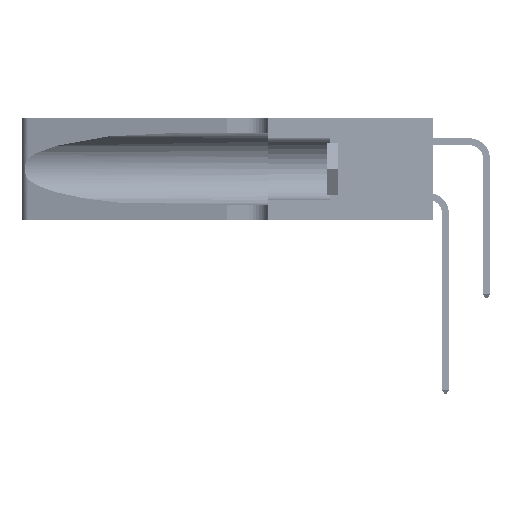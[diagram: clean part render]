
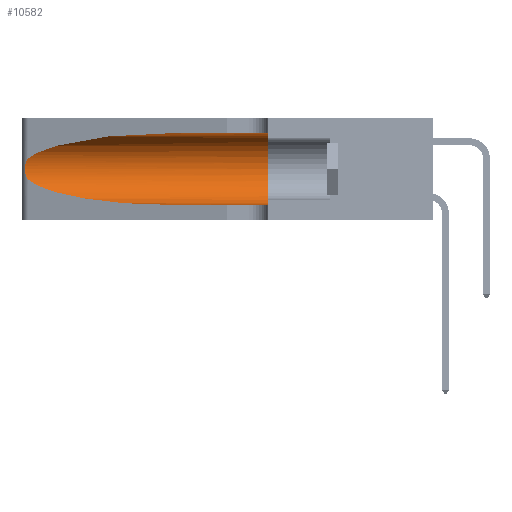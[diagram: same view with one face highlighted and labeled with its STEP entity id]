
A CAD part, left-side view. The second image highlights one B-rep face of the part: STEP entity #10582.
In plain terms, the highlighted cylindrical face has radius 3.308 mm (diameter 6.617 mm), a partial arc.
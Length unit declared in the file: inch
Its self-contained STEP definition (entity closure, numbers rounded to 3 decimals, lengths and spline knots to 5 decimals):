
#1970 = CARTESIAN_POINT ( 'NONE',  ( 0.1305, 1.61858, 0.05475 ) ) ;
#4043 = CARTESIAN_POINT ( 'NONE',  ( 0.25854, 1.2359, 0.20912 ) ) ;
#6457 = CARTESIAN_POINT ( 'NONE',  ( 0.1305, 0.72297, 0.31525 ) ) ;
#7393 = VECTOR ( 'NONE', #19006, 39.37008 ) ;
#8060 = FACE_OUTER_BOUND ( 'NONE', #13091, .T. ) ;
#8213 = CARTESIAN_POINT ( 'NONE',  ( 0.26075, 1.23896, 0.19203 ) ) ;
#8369 = ORIENTED_EDGE ( 'NONE', *, *, #14442, .T. ) ;
#10315 = CARTESIAN_POINT ( 'NONE',  ( 0.1305, 0.35, 0.185 ) ) ;
#10350 = DIRECTION ( 'NONE',  ( 0., -1., 0. ) ) ;
#10582 = ADVANCED_FACE ( 'NONE', ( #8060 ), #17905, .F. ) ;
#11391 = ORIENTED_EDGE ( 'NONE', *, *, #20961, .F. ) ;
#12233 = CARTESIAN_POINT ( 'NONE',  ( 0.25487, 1.22718, 0.22369 ) ) ;
#12414 = CARTESIAN_POINT ( 'NONE',  ( 0.26017, 1.23833, 0.17102 ) ) ;
#12595 = CARTESIAN_POINT ( 'NONE',  ( 0.1305, 0.72297, 0.31525 ) ) ;
#13091 = EDGE_LOOP ( 'NONE', ( #46398, #51525, #8369, #25007, #44437, #11391 ) ) ;
#14442 = EDGE_CURVE ( 'NONE', #21079, #15864, #38820, .T. ) ;
#14537 = DIRECTION ( 'NONE',  ( 0., 0., 1. ) ) ;
#15864 = VERTEX_POINT ( 'NONE', #43394 ) ;
#16449 = CARTESIAN_POINT ( 'NONE',  ( 0.25555, 1.22994, 0.2215 ) ) ;
#16636 = CARTESIAN_POINT ( 'NONE',  ( 0.25789, 1.23486, 0.15765 ) ) ;
#16812 = CARTESIAN_POINT ( 'NONE',  ( 0.2373, 1.15595, 0.28018 ) ) ;
#16832 = CARTESIAN_POINT ( 'NONE',  ( 0.25487, 1.22718, 0.22369 ) ) ;
#17185 = LINE ( 'NONE', #52155, #7393 ) ;
#17412 = EDGE_CURVE ( 'NONE', #44796, #41826, #27427, .T. ) ;
#17905 = CYLINDRICAL_SURFACE ( 'NONE', #35872, 0.13025 ) ;
#19006 = DIRECTION ( 'NONE',  ( 0., -1., 0. ) ) ;
#19559 =( BOUNDED_CURVE ( )  B_SPLINE_CURVE ( 3, ( #12595, #37519, #16812, #45783 ),
 .UNSPECIFIED., .F., .T. ) 
 B_SPLINE_CURVE_WITH_KNOTS ( ( 4, 4 ),
 ( 1.5708, 2.84003 ),
 .UNSPECIFIED. ) 
 CURVE ( )  GEOMETRIC_REPRESENTATION_ITEM ( )  RATIONAL_B_SPLINE_CURVE ( ( 1., 0.87, 0.87, 1. ) ) 
 REPRESENTATION_ITEM ( '' )  );
#20548 = CARTESIAN_POINT ( 'NONE',  ( 0.1305, 0.35, 0.05475 ) ) ;
#20565 = EDGE_CURVE ( 'NONE', #43574, #38137, #19559, .T. ) ;
#20851 = LINE ( 'NONE', #1970, #52433 ) ;
#20856 = CARTESIAN_POINT ( 'NONE',  ( 0.25555, 1.22993, 0.14849 ) ) ;
#20961 = EDGE_CURVE ( 'NONE', #43574, #44796, #17185, .T. ) ;
#21079 = VERTEX_POINT ( 'NONE', #36593 ) ;
#22008 = CARTESIAN_POINT ( 'NONE',  ( 0.25487, 1.22718, 0.14631 ) ) ;
#22190 = CARTESIAN_POINT ( 'NONE',  ( 0.18966, 0.96281, 0.05475 ) ) ;
#25007 = ORIENTED_EDGE ( 'NONE', *, *, #36453, .T. ) ;
#27389 = AXIS2_PLACEMENT_3D ( 'NONE', #10315, #39422, #14537 ) ;
#27427 = CIRCLE ( 'NONE', #27389, 0.13025 ) ;
#29043 = CARTESIAN_POINT ( 'NONE',  ( 0.25787, 1.23484, 0.2124 ) ) ;
#30854 = B_SPLINE_CURVE_WITH_KNOTS ( 'NONE', 3,
 ( #12233, #16449, #53642, #29043, #4043, #33190, #8213, #37346, #12414, #41479, #16636, #45599, #20856, #49695 ),
 .UNSPECIFIED., .F., .F.,
 ( 4, 2, 2, 2, 2, 2, 4 ),
 ( 0., 0.00027, 0.00053, 0.00107, 0.0016, 0.00187, 0.00214 ),
 .UNSPECIFIED. ) ;
#33190 = CARTESIAN_POINT ( 'NONE',  ( 0.26018, 1.23835, 0.19895 ) ) ;
#34096 = DIRECTION ( 'NONE',  ( 0., -1., 0. ) ) ;
#35872 = AXIS2_PLACEMENT_3D ( 'NONE', #50598, #34096, #38246 ) ;
#36453 = EDGE_CURVE ( 'NONE', #15864, #41826, #20851, .T. ) ;
#36593 = CARTESIAN_POINT ( 'NONE',  ( 0.25487, 1.22718, 0.14631 ) ) ;
#37346 = CARTESIAN_POINT ( 'NONE',  ( 0.26075, 1.23896, 0.178 ) ) ;
#37519 = CARTESIAN_POINT ( 'NONE',  ( 0.18966, 0.96281, 0.31525 ) ) ;
#38137 = VERTEX_POINT ( 'NONE', #16832 ) ;
#38246 = DIRECTION ( 'NONE',  ( 0., 0., -1. ) ) ;
#38820 =( BOUNDED_CURVE ( )  B_SPLINE_CURVE ( 3, ( #22008, #46921, #22190, #50997 ),
 .UNSPECIFIED., .F., .T. ) 
 B_SPLINE_CURVE_WITH_KNOTS ( ( 4, 4 ),
 ( 3.44316, 4.71239 ),
 .UNSPECIFIED. ) 
 CURVE ( )  GEOMETRIC_REPRESENTATION_ITEM ( )  RATIONAL_B_SPLINE_CURVE ( ( 1., 0.87, 0.87, 1. ) ) 
 REPRESENTATION_ITEM ( '' )  );
#39422 = DIRECTION ( 'NONE',  ( 0., 1., 0. ) ) ;
#41479 = CARTESIAN_POINT ( 'NONE',  ( 0.25856, 1.23593, 0.16098 ) ) ;
#41826 = VERTEX_POINT ( 'NONE', #20548 ) ;
#43394 = CARTESIAN_POINT ( 'NONE',  ( 0.1305, 0.72297, 0.05475 ) ) ;
#43574 = VERTEX_POINT ( 'NONE', #6457 ) ;
#44437 = ORIENTED_EDGE ( 'NONE', *, *, #17412, .F. ) ;
#44796 = VERTEX_POINT ( 'NONE', #47277 ) ;
#45599 = CARTESIAN_POINT ( 'NONE',  ( 0.25639, 1.23186, 0.15144 ) ) ;
#45783 = CARTESIAN_POINT ( 'NONE',  ( 0.25487, 1.22718, 0.22369 ) ) ;
#46398 = ORIENTED_EDGE ( 'NONE', *, *, #20565, .T. ) ;
#46921 = CARTESIAN_POINT ( 'NONE',  ( 0.2373, 1.15595, 0.08982 ) ) ;
#47277 = CARTESIAN_POINT ( 'NONE',  ( 0.1305, 0.35, 0.31525 ) ) ;
#49695 = CARTESIAN_POINT ( 'NONE',  ( 0.25487, 1.22718, 0.14631 ) ) ;
#50598 = CARTESIAN_POINT ( 'NONE',  ( 0.1305, 1.61858, 0.185 ) ) ;
#50831 = EDGE_CURVE ( 'NONE', #38137, #21079, #30854, .T. ) ;
#50997 = CARTESIAN_POINT ( 'NONE',  ( 0.1305, 0.72297, 0.05475 ) ) ;
#51525 = ORIENTED_EDGE ( 'NONE', *, *, #50831, .T. ) ;
#52155 = CARTESIAN_POINT ( 'NONE',  ( 0.1305, 1.61858, 0.31525 ) ) ;
#52433 = VECTOR ( 'NONE', #10350, 39.37008 ) ;
#53642 = CARTESIAN_POINT ( 'NONE',  ( 0.25639, 1.23184, 0.21858 ) ) ;
